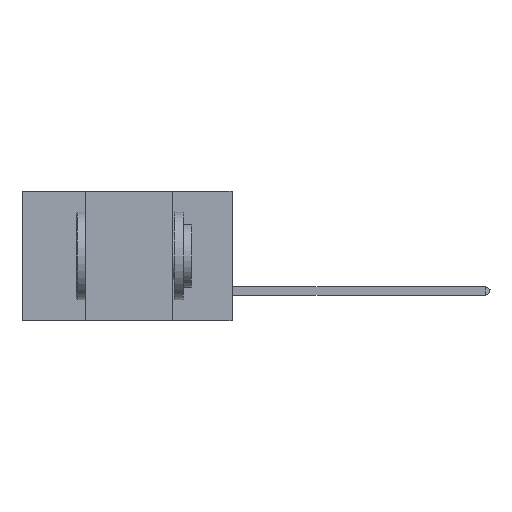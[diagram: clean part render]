
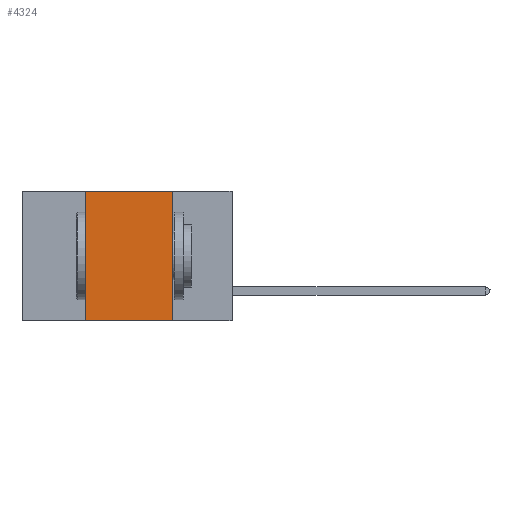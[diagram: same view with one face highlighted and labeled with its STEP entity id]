
A CAD part, left-side view. The second image highlights one B-rep face of the part: STEP entity #4324.
In plain terms, the highlighted planar face has unit normal (-1, 0, 0).
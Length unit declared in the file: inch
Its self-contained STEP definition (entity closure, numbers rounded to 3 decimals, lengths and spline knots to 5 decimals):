
#6 = VECTOR ( 'NONE', #302, 39.37008 ) ;
#62 = PLANE ( 'NONE',  #2569 ) ;
#171 = FACE_OUTER_BOUND ( 'NONE', #11689, .T. ) ;
#302 = DIRECTION ( 'NONE',  ( 0., 0., -1. ) ) ;
#386 = VERTEX_POINT ( 'NONE', #4935 ) ;
#992 = DIRECTION ( 'NONE',  ( 0., 0., -1. ) ) ;
#1252 = VERTEX_POINT ( 'NONE', #8366 ) ;
#1867 = CARTESIAN_POINT ( 'NONE',  ( 0., 0.6, 0. ) ) ;
#2436 = ORIENTED_EDGE ( 'NONE', *, *, #7617, .F. ) ;
#2569 = AXIS2_PLACEMENT_3D ( 'NONE', #5505, #6542, #992 ) ;
#2913 = VERTEX_POINT ( 'NONE', #6953 ) ;
#3321 = CARTESIAN_POINT ( 'NONE',  ( 0., 0.6, -0.37 ) ) ;
#3404 = ORIENTED_EDGE ( 'NONE', *, *, #4034, .T. ) ;
#3514 = LINE ( 'NONE', #3321, #5542 ) ;
#3785 = DIRECTION ( 'NONE',  ( 0., -1., 0. ) ) ;
#3814 = CARTESIAN_POINT ( 'NONE',  ( 0., 0.42, -0.37 ) ) ;
#3986 = CARTESIAN_POINT ( 'NONE',  ( 0., 0.17, 0. ) ) ;
#4034 = EDGE_CURVE ( 'NONE', #4680, #386, #3514, .T. ) ;
#4141 = ORIENTED_EDGE ( 'NONE', *, *, #6269, .F. ) ;
#4324 = ADVANCED_FACE ( 'NONE', ( #171 ), #62, .F. ) ;
#4680 = VERTEX_POINT ( 'NONE', #3814 ) ;
#4935 = CARTESIAN_POINT ( 'NONE',  ( 0., 0.17, -0.37 ) ) ;
#5021 = DIRECTION ( 'NONE',  ( 0., 0., 1. ) ) ;
#5505 = CARTESIAN_POINT ( 'NONE',  ( 0., 0.6, 0. ) ) ;
#5542 = VECTOR ( 'NONE', #9726, 39.37008 ) ;
#5729 = VECTOR ( 'NONE', #3785, 39.37008 ) ;
#6269 = EDGE_CURVE ( 'NONE', #2913, #386, #7404, .T. ) ;
#6542 = DIRECTION ( 'NONE',  ( 1., 0., 0. ) ) ;
#6953 = CARTESIAN_POINT ( 'NONE',  ( 0., 0.17, 0. ) ) ;
#7321 = LINE ( 'NONE', #1867, #5729 ) ;
#7404 = LINE ( 'NONE', #3986, #6 ) ;
#7617 = EDGE_CURVE ( 'NONE', #4680, #1252, #8080, .T. ) ;
#8080 = LINE ( 'NONE', #11524, #8655 ) ;
#8366 = CARTESIAN_POINT ( 'NONE',  ( 0., 0.42, 0. ) ) ;
#8655 = VECTOR ( 'NONE', #5021, 39.37008 ) ;
#9407 = ORIENTED_EDGE ( 'NONE', *, *, #11760, .F. ) ;
#9726 = DIRECTION ( 'NONE',  ( 0., -1., 0. ) ) ;
#11524 = CARTESIAN_POINT ( 'NONE',  ( 0., 0.42, 0. ) ) ;
#11689 = EDGE_LOOP ( 'NONE', ( #4141, #9407, #2436, #3404 ) ) ;
#11760 = EDGE_CURVE ( 'NONE', #1252, #2913, #7321, .T. ) ;
